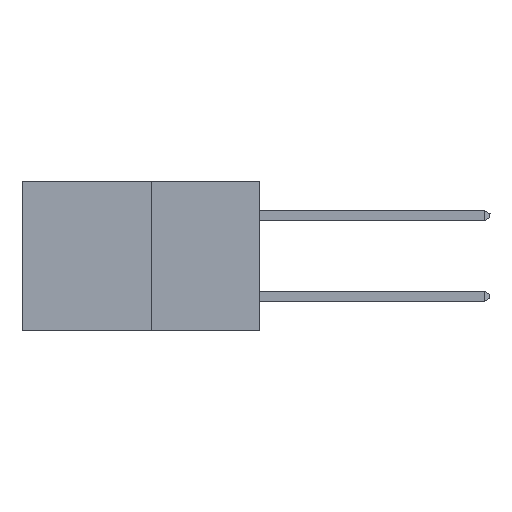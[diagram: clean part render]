
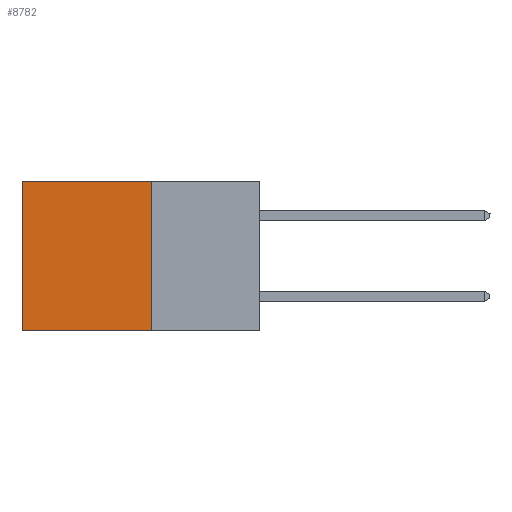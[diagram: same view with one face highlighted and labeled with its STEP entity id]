
A CAD part, left-side view. The second image highlights one B-rep face of the part: STEP entity #8782.
In plain terms, the highlighted planar face has unit normal (-1, 0, 0).
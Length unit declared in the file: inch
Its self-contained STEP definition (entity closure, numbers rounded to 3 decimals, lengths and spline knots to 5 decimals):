
#32 = VERTEX_POINT ( 'NONE', #2347 ) ;
#322 = CARTESIAN_POINT ( 'NONE',  ( 0.277, 0.59, -0.37 ) ) ;
#497 = EDGE_CURVE ( 'NONE', #4529, #2751, #4436, .T. ) ;
#1177 = CARTESIAN_POINT ( 'NONE',  ( 0.277, 0.59, 0. ) ) ;
#1319 = DIRECTION ( 'NONE',  ( 0., 0., -1. ) ) ;
#1481 = DIRECTION ( 'NONE',  ( 0., 1., 0. ) ) ;
#1511 = CARTESIAN_POINT ( 'NONE',  ( 0.277, 0.27, 0. ) ) ;
#1842 = EDGE_CURVE ( 'NONE', #32, #2751, #9647, .T. ) ;
#2347 = CARTESIAN_POINT ( 'NONE',  ( 0.277, 0.27, -0.37 ) ) ;
#2751 = VERTEX_POINT ( 'NONE', #322 ) ;
#3250 = DIRECTION ( 'NONE',  ( 0., 0., -1. ) ) ;
#3265 = DIRECTION ( 'NONE',  ( 1., 0., 0. ) ) ;
#3279 = CARTESIAN_POINT ( 'NONE',  ( 0.277, 0.27, -0.37 ) ) ;
#3290 = PLANE ( 'NONE',  #6976 ) ;
#4436 = LINE ( 'NONE', #8457, #12873 ) ;
#4529 = VERTEX_POINT ( 'NONE', #1177 ) ;
#5238 = EDGE_LOOP ( 'NONE', ( #6825, #7517, #8148, #5634 ) ) ;
#5375 = VERTEX_POINT ( 'NONE', #11651 ) ;
#5634 = ORIENTED_EDGE ( 'NONE', *, *, #11600, .T. ) ;
#6044 = LINE ( 'NONE', #11550, #8542 ) ;
#6825 = ORIENTED_EDGE ( 'NONE', *, *, #497, .T. ) ;
#6908 = VECTOR ( 'NONE', #9318, 39.37008 ) ;
#6976 = AXIS2_PLACEMENT_3D ( 'NONE', #3279, #3265, #3250 ) ;
#7517 = ORIENTED_EDGE ( 'NONE', *, *, #1842, .F. ) ;
#8148 = ORIENTED_EDGE ( 'NONE', *, *, #12053, .F. ) ;
#8312 = DIRECTION ( 'NONE',  ( 0., 0., -1. ) ) ;
#8457 = CARTESIAN_POINT ( 'NONE',  ( 0.277, 0.59, -0.37 ) ) ;
#8542 = VECTOR ( 'NONE', #1319, 39.37008 ) ;
#8782 = ADVANCED_FACE ( 'NONE', ( #10827 ), #3290, .F. ) ;
#9147 = LINE ( 'NONE', #1511, #11517 ) ;
#9318 = DIRECTION ( 'NONE',  ( 0., 1., 0. ) ) ;
#9647 = LINE ( 'NONE', #10782, #6908 ) ;
#10782 = CARTESIAN_POINT ( 'NONE',  ( 0.277, 0.27, -0.37 ) ) ;
#10827 = FACE_OUTER_BOUND ( 'NONE', #5238, .T. ) ;
#11517 = VECTOR ( 'NONE', #1481, 39.37008 ) ;
#11550 = CARTESIAN_POINT ( 'NONE',  ( 0.277, 0.27, -0.37 ) ) ;
#11600 = EDGE_CURVE ( 'NONE', #5375, #4529, #9147, .T. ) ;
#11651 = CARTESIAN_POINT ( 'NONE',  ( 0.277, 0.27, 0. ) ) ;
#12053 = EDGE_CURVE ( 'NONE', #5375, #32, #6044, .T. ) ;
#12873 = VECTOR ( 'NONE', #8312, 39.37008 ) ;
